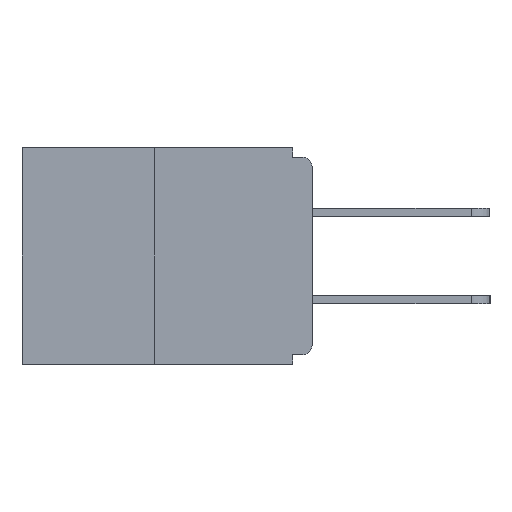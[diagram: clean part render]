
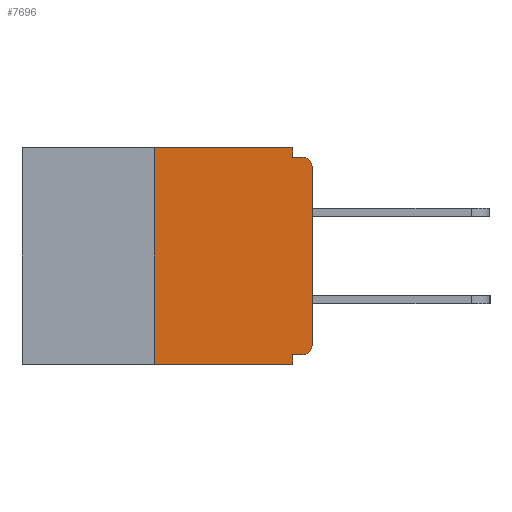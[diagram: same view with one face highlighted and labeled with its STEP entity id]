
A CAD part, left-side view. The second image highlights one B-rep face of the part: STEP entity #7696.
In plain terms, the highlighted planar face has unit normal (-1, 0, 0).
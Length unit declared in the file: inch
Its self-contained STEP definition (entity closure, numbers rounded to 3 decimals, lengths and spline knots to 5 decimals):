
#307 = CARTESIAN_POINT ( 'NONE',  ( 0., 0.015, -0.03 ) ) ;
#367 = LINE ( 'NONE', #15062, #16721 ) ;
#570 = CARTESIAN_POINT ( 'NONE',  ( 0., 0.015, -0.328 ) ) ;
#723 = CARTESIAN_POINT ( 'NONE',  ( 0., 0.25, 0. ) ) ;
#769 = VERTEX_POINT ( 'NONE', #4600 ) ;
#920 = CARTESIAN_POINT ( 'NONE',  ( 0., 0.015, -0.015 ) ) ;
#1405 = ORIENTED_EDGE ( 'NONE', *, *, #8620, .T. ) ;
#1448 = DIRECTION ( 'NONE',  ( 0., -1., 0. ) ) ;
#1462 = FACE_OUTER_BOUND ( 'NONE', #11882, .T. ) ;
#2026 = CARTESIAN_POINT ( 'NONE',  ( 0., 0.25, -0.343 ) ) ;
#2396 = CARTESIAN_POINT ( 'NONE',  ( 0., 0.25, 0. ) ) ;
#2414 = AXIS2_PLACEMENT_3D ( 'NONE', #307, #12094, #2750 ) ;
#2538 = DIRECTION ( 'NONE',  ( 0., 0., -1. ) ) ;
#2750 = DIRECTION ( 'NONE',  ( 0., 0., -1. ) ) ;
#3664 = LINE ( 'NONE', #13366, #4912 ) ;
#4600 = CARTESIAN_POINT ( 'NONE',  ( 0., 0.031, 0. ) ) ;
#4675 = DIRECTION ( 'NONE',  ( 0., -1., 0. ) ) ;
#4686 = EDGE_CURVE ( 'NONE', #14815, #769, #5721, .T. ) ;
#4879 = DIRECTION ( 'NONE',  ( 0., 0., -1. ) ) ;
#4912 = VECTOR ( 'NONE', #2538, 39.37008 ) ;
#5506 = ORIENTED_EDGE ( 'NONE', *, *, #9876, .T. ) ;
#5512 = DIRECTION ( 'NONE',  ( 0., -1., 0. ) ) ;
#5628 = DIRECTION ( 'NONE',  ( 0., 0., -1. ) ) ;
#5721 = LINE ( 'NONE', #9623, #6686 ) ;
#5865 = VECTOR ( 'NONE', #4675, 39.37008 ) ;
#6114 = LINE ( 'NONE', #20320, #15275 ) ;
#6339 = CARTESIAN_POINT ( 'NONE',  ( 0., 0.031, -0.328 ) ) ;
#6369 = LINE ( 'NONE', #8809, #12858 ) ;
#6686 = VECTOR ( 'NONE', #1448, 39.37008 ) ;
#7201 = DIRECTION ( 'NONE',  ( 0., 1., 0. ) ) ;
#7466 = PLANE ( 'NONE',  #19608 ) ;
#7696 = ADVANCED_FACE ( 'NONE', ( #1462 ), #7466, .F. ) ;
#7760 = CARTESIAN_POINT ( 'NONE',  ( 0., 0., 0. ) ) ;
#8171 = EDGE_CURVE ( 'NONE', #14314, #14815, #19507, .T. ) ;
#8620 = EDGE_CURVE ( 'NONE', #14314, #15580, #6114, .T. ) ;
#8689 = EDGE_CURVE ( 'NONE', #16900, #14861, #10609, .T. ) ;
#8809 = CARTESIAN_POINT ( 'NONE',  ( 0., 0.031, -0.343 ) ) ;
#9130 = VERTEX_POINT ( 'NONE', #570 ) ;
#9200 = CARTESIAN_POINT ( 'NONE',  ( 0., 0.46, 0. ) ) ;
#9362 = DIRECTION ( 'NONE',  ( 0., 0., 1. ) ) ;
#9416 = CARTESIAN_POINT ( 'NONE',  ( 0., 0., -0.015 ) ) ;
#9623 = CARTESIAN_POINT ( 'NONE',  ( 0., 0.46, 0. ) ) ;
#9876 = EDGE_CURVE ( 'NONE', #16790, #14861, #17675, .T. ) ;
#10379 = VECTOR ( 'NONE', #15516, 39.37008 ) ;
#10609 = LINE ( 'NONE', #9416, #5865 ) ;
#10661 = DIRECTION ( 'NONE',  ( 1., 0., 0. ) ) ;
#10923 = EDGE_CURVE ( 'NONE', #19647, #16790, #11026, .T. ) ;
#11026 = LINE ( 'NONE', #7760, #19881 ) ;
#11167 = ORIENTED_EDGE ( 'NONE', *, *, #8689, .F. ) ;
#11270 = CARTESIAN_POINT ( 'NONE',  ( 0., 0.015, -0.313 ) ) ;
#11411 = DIRECTION ( 'NONE',  ( -1., 0., 0. ) ) ;
#11709 = CARTESIAN_POINT ( 'NONE',  ( 0., 0.031, -0.343 ) ) ;
#11882 = EDGE_LOOP ( 'NONE', ( #14372, #12963, #1405, #13673, #12360, #14247, #15059, #5506, #11167, #16579 ) ) ;
#12094 = DIRECTION ( 'NONE',  ( -1., 0., 0. ) ) ;
#12360 = ORIENTED_EDGE ( 'NONE', *, *, #16051, .F. ) ;
#12858 = VECTOR ( 'NONE', #5628, 39.37008 ) ;
#12963 = ORIENTED_EDGE ( 'NONE', *, *, #8171, .F. ) ;
#13140 = AXIS2_PLACEMENT_3D ( 'NONE', #11270, #11411, #4879 ) ;
#13219 = CIRCLE ( 'NONE', #13140, 0.015 ) ;
#13366 = CARTESIAN_POINT ( 'NONE',  ( 0., 0.031, 0. ) ) ;
#13473 = VERTEX_POINT ( 'NONE', #6339 ) ;
#13567 = CARTESIAN_POINT ( 'NONE',  ( 0., 0.031, -0.015 ) ) ;
#13673 = ORIENTED_EDGE ( 'NONE', *, *, #14377, .F. ) ;
#13906 = EDGE_CURVE ( 'NONE', #769, #16900, #3664, .T. ) ;
#14247 = ORIENTED_EDGE ( 'NONE', *, *, #17818, .T. ) ;
#14314 = VERTEX_POINT ( 'NONE', #2026 ) ;
#14372 = ORIENTED_EDGE ( 'NONE', *, *, #4686, .F. ) ;
#14377 = EDGE_CURVE ( 'NONE', #13473, #15580, #6369, .T. ) ;
#14815 = VERTEX_POINT ( 'NONE', #2396 ) ;
#14861 = VERTEX_POINT ( 'NONE', #920 ) ;
#15059 = ORIENTED_EDGE ( 'NONE', *, *, #10923, .T. ) ;
#15062 = CARTESIAN_POINT ( 'NONE',  ( 0., 0., -0.328 ) ) ;
#15275 = VECTOR ( 'NONE', #5512, 39.37008 ) ;
#15516 = DIRECTION ( 'NONE',  ( 0., 0., 1. ) ) ;
#15580 = VERTEX_POINT ( 'NONE', #11709 ) ;
#16051 = EDGE_CURVE ( 'NONE', #9130, #13473, #367, .T. ) ;
#16579 = ORIENTED_EDGE ( 'NONE', *, *, #13906, .F. ) ;
#16721 = VECTOR ( 'NONE', #7201, 39.37008 ) ;
#16790 = VERTEX_POINT ( 'NONE', #19338 ) ;
#16900 = VERTEX_POINT ( 'NONE', #13567 ) ;
#16981 = DIRECTION ( 'NONE',  ( 0., 0., -1. ) ) ;
#17675 = CIRCLE ( 'NONE', #2414, 0.015 ) ;
#17818 = EDGE_CURVE ( 'NONE', #9130, #19647, #13219, .T. ) ;
#17852 = CARTESIAN_POINT ( 'NONE',  ( 0., 0., -0.313 ) ) ;
#19338 = CARTESIAN_POINT ( 'NONE',  ( 0., 0., -0.03 ) ) ;
#19507 = LINE ( 'NONE', #723, #10379 ) ;
#19608 = AXIS2_PLACEMENT_3D ( 'NONE', #9200, #10661, #16981 ) ;
#19647 = VERTEX_POINT ( 'NONE', #17852 ) ;
#19881 = VECTOR ( 'NONE', #9362, 39.37008 ) ;
#20320 = CARTESIAN_POINT ( 'NONE',  ( 0., 0.46, -0.343 ) ) ;
